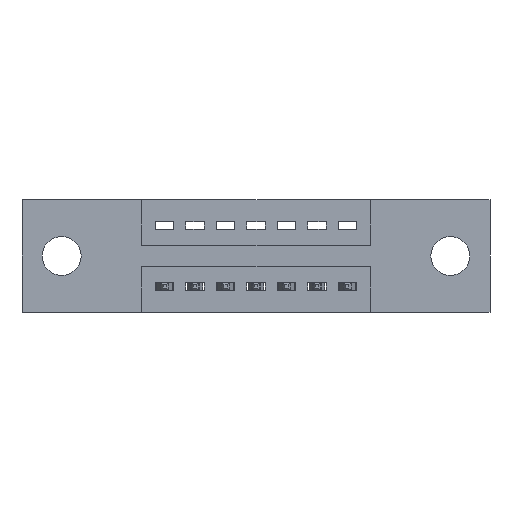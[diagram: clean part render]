
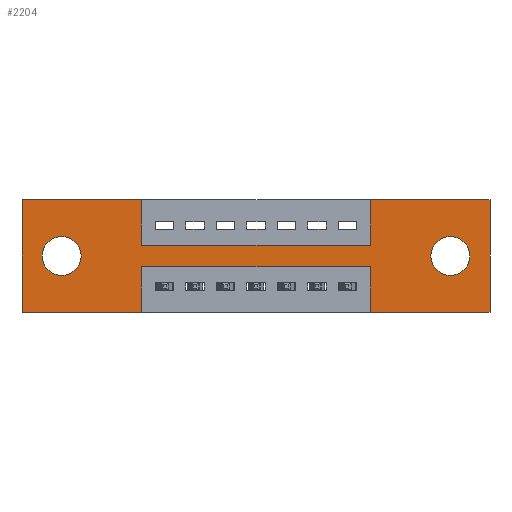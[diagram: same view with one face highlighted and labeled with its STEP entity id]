
A CAD part, front view. The second image highlights one B-rep face of the part: STEP entity #2204.
In plain terms, the highlighted planar face has unit normal (0, -1, 0).
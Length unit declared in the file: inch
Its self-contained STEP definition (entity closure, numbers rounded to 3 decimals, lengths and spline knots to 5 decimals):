
#175 = CARTESIAN_POINT ( 'NONE',  ( 0., 0., -0.37 ) ) ;
#200 = CARTESIAN_POINT ( 'NONE',  ( 0., 0., 0. ) ) ;
#263 = CARTESIAN_POINT ( 'NONE',  ( 0.3925, 0., -0.37 ) ) ;
#467 = CARTESIAN_POINT ( 'NONE',  ( 0., 0., -0.37 ) ) ;
#705 = VERTEX_POINT ( 'NONE', #1946 ) ;
#754 = EDGE_CURVE ( 'NONE', #2903, #5305, #3198, .T. ) ;
#755 = DIRECTION ( 'NONE',  ( 0., 0., -1. ) ) ;
#815 = ORIENTED_EDGE ( 'NONE', *, *, #8343, .F. ) ;
#854 = EDGE_CURVE ( 'NONE', #8996, #8657, #7049, .T. ) ;
#1015 = FACE_BOUND ( 'NONE', #9133, .T. ) ;
#1070 = CARTESIAN_POINT ( 'NONE',  ( 1.1425, 0., -0.22 ) ) ;
#1075 = AXIS2_PLACEMENT_3D ( 'NONE', #2217, #7555, #5308 ) ;
#1172 = ORIENTED_EDGE ( 'NONE', *, *, #2373, .F. ) ;
#1248 = VERTEX_POINT ( 'NONE', #8144 ) ;
#1264 = EDGE_CURVE ( 'NONE', #8352, #7169, #3689, .T. ) ;
#1525 = CIRCLE ( 'NONE', #3843, 0.064 ) ;
#1534 = DIRECTION ( 'NONE',  ( 0., 0., 1. ) ) ;
#1598 = LINE ( 'NONE', #7795, #9582 ) ;
#1729 = AXIS2_PLACEMENT_3D ( 'NONE', #3698, #6703, #9168 ) ;
#1784 = VECTOR ( 'NONE', #7000, 39.37008 ) ;
#1946 = CARTESIAN_POINT ( 'NONE',  ( 1.1425, 0., -0.15 ) ) ;
#2011 = DIRECTION ( 'NONE',  ( 1., 0., 0. ) ) ;
#2152 = PLANE ( 'NONE',  #1075 ) ;
#2199 = CARTESIAN_POINT ( 'NONE',  ( 1.405, 0., -0.121 ) ) ;
#2204 = ADVANCED_FACE ( 'NONE', ( #6083, #1015, #8509 ), #2152, .T. ) ;
#2217 = CARTESIAN_POINT ( 'NONE',  ( 0., 0., -0.37 ) ) ;
#2307 = EDGE_CURVE ( 'NONE', #7169, #2903, #1598, .T. ) ;
#2367 = DIRECTION ( 'NONE',  ( 0., 0., -1. ) ) ;
#2373 = EDGE_CURVE ( 'NONE', #5305, #9521, #9115, .T. ) ;
#2410 = EDGE_LOOP ( 'NONE', ( #6445, #5243, #4363, #8987, #815, #9466, #6175, #9647, #1172, #7229, #9069, #9988 ) ) ;
#2497 = CARTESIAN_POINT ( 'NONE',  ( 1.535, 0., 0. ) ) ;
#2546 = CARTESIAN_POINT ( 'NONE',  ( 1.405, 0., -0.249 ) ) ;
#2813 = CARTESIAN_POINT ( 'NONE',  ( 0.3925, 0., -0.37 ) ) ;
#2903 = VERTEX_POINT ( 'NONE', #9657 ) ;
#2953 = VERTEX_POINT ( 'NONE', #5676 ) ;
#3198 = LINE ( 'NONE', #3631, #4995 ) ;
#3357 = VERTEX_POINT ( 'NONE', #6620 ) ;
#3557 = CARTESIAN_POINT ( 'NONE',  ( 0.3925, 0., -0.22 ) ) ;
#3631 = CARTESIAN_POINT ( 'NONE',  ( 0., 0., 0. ) ) ;
#3689 = LINE ( 'NONE', #467, #6296 ) ;
#3698 = CARTESIAN_POINT ( 'NONE',  ( 0.13, 0., -0.185 ) ) ;
#3806 = EDGE_CURVE ( 'NONE', #2953, #8352, #5798, .T. ) ;
#3830 = CIRCLE ( 'NONE', #7728, 0.064 ) ;
#3843 = AXIS2_PLACEMENT_3D ( 'NONE', #6954, #7621, #755 ) ;
#3869 = LINE ( 'NONE', #5439, #1784 ) ;
#3884 = CARTESIAN_POINT ( 'NONE',  ( 1.535, 0., -0.37 ) ) ;
#4083 = VECTOR ( 'NONE', #8032, 39.37008 ) ;
#4292 = ORIENTED_EDGE ( 'NONE', *, *, #5644, .T. ) ;
#4363 = ORIENTED_EDGE ( 'NONE', *, *, #8855, .F. ) ;
#4454 = LINE ( 'NONE', #3557, #6737 ) ;
#4538 = DIRECTION ( 'NONE',  ( 1., 0., 0. ) ) ;
#4678 = DIRECTION ( 'NONE',  ( 0., 0., -1. ) ) ;
#4696 = EDGE_CURVE ( 'NONE', #9521, #705, #9186, .T. ) ;
#4995 = VECTOR ( 'NONE', #2011, 39.37008 ) ;
#5022 = ORIENTED_EDGE ( 'NONE', *, *, #9738, .T. ) ;
#5105 = DIRECTION ( 'NONE',  ( 0., 0., 1. ) ) ;
#5137 = DIRECTION ( 'NONE',  ( -1., 0., 0. ) ) ;
#5243 = ORIENTED_EDGE ( 'NONE', *, *, #7178, .F. ) ;
#5276 = CARTESIAN_POINT ( 'NONE',  ( 0.13, 0., -0.249 ) ) ;
#5305 = VERTEX_POINT ( 'NONE', #8476 ) ;
#5308 = DIRECTION ( 'NONE',  ( 0., 0., -1. ) ) ;
#5342 = EDGE_LOOP ( 'NONE', ( #9038, #4292 ) ) ;
#5385 = VERTEX_POINT ( 'NONE', #3884 ) ;
#5439 = CARTESIAN_POINT ( 'NONE',  ( 0., 0., -0.37 ) ) ;
#5533 = DIRECTION ( 'NONE',  ( 0., 1., 0. ) ) ;
#5644 = EDGE_CURVE ( 'NONE', #7117, #7827, #9764, .T. ) ;
#5646 = EDGE_CURVE ( 'NONE', #7827, #7117, #1525, .T. ) ;
#5676 = CARTESIAN_POINT ( 'NONE',  ( 0.3925, 0., -0.22 ) ) ;
#5688 = VERTEX_POINT ( 'NONE', #8698 ) ;
#5798 = LINE ( 'NONE', #2813, #6386 ) ;
#5833 = EDGE_CURVE ( 'NONE', #5385, #1248, #3869, .T. ) ;
#5989 = VERTEX_POINT ( 'NONE', #1070 ) ;
#6083 = FACE_BOUND ( 'NONE', #5342, .T. ) ;
#6175 = ORIENTED_EDGE ( 'NONE', *, *, #8043, .F. ) ;
#6296 = VECTOR ( 'NONE', #5137, 39.37008 ) ;
#6386 = VECTOR ( 'NONE', #9870, 39.37008 ) ;
#6388 = AXIS2_PLACEMENT_3D ( 'NONE', #9788, #5533, #8443 ) ;
#6427 = CARTESIAN_POINT ( 'NONE',  ( 0.3925, 0., -0.15 ) ) ;
#6445 = ORIENTED_EDGE ( 'NONE', *, *, #3806, .F. ) ;
#6493 = CARTESIAN_POINT ( 'NONE',  ( 0.13, 0., -0.185 ) ) ;
#6524 = CARTESIAN_POINT ( 'NONE',  ( 1.1425, 0., 0. ) ) ;
#6620 = CARTESIAN_POINT ( 'NONE',  ( 1.535, 0., 0. ) ) ;
#6703 = DIRECTION ( 'NONE',  ( 0., 1., 0. ) ) ;
#6737 = VECTOR ( 'NONE', #8962, 39.37008 ) ;
#6921 = CARTESIAN_POINT ( 'NONE',  ( 1.1425, 0., -0.37 ) ) ;
#6928 = LINE ( 'NONE', #6921, #9862 ) ;
#6954 = CARTESIAN_POINT ( 'NONE',  ( 1.405, 0., -0.185 ) ) ;
#7000 = DIRECTION ( 'NONE',  ( -1., 0., 0. ) ) ;
#7049 = CIRCLE ( 'NONE', #1729, 0.064 ) ;
#7060 = CARTESIAN_POINT ( 'NONE',  ( 0.3925, 0., 0. ) ) ;
#7117 = VERTEX_POINT ( 'NONE', #2546 ) ;
#7169 = VERTEX_POINT ( 'NONE', #175 ) ;
#7178 = EDGE_CURVE ( 'NONE', #5989, #2953, #4454, .T. ) ;
#7191 = VECTOR ( 'NONE', #2367, 39.37008 ) ;
#7229 = ORIENTED_EDGE ( 'NONE', *, *, #754, .F. ) ;
#7555 = DIRECTION ( 'NONE',  ( 0., -1., 0. ) ) ;
#7621 = DIRECTION ( 'NONE',  ( 0., 1., 0. ) ) ;
#7728 = AXIS2_PLACEMENT_3D ( 'NONE', #6493, #8081, #5105 ) ;
#7742 = ORIENTED_EDGE ( 'NONE', *, *, #854, .T. ) ;
#7758 = EDGE_CURVE ( 'NONE', #5688, #3357, #8449, .T. ) ;
#7795 = CARTESIAN_POINT ( 'NONE',  ( 0., 0., 0. ) ) ;
#7827 = VERTEX_POINT ( 'NONE', #2199 ) ;
#7830 = LINE ( 'NONE', #6524, #8794 ) ;
#8032 = DIRECTION ( 'NONE',  ( 1., 0., 0. ) ) ;
#8043 = EDGE_CURVE ( 'NONE', #705, #5688, #7830, .T. ) ;
#8081 = DIRECTION ( 'NONE',  ( 0., 1., 0. ) ) ;
#8144 = CARTESIAN_POINT ( 'NONE',  ( 1.1425, 0., -0.37 ) ) ;
#8343 = EDGE_CURVE ( 'NONE', #3357, #5385, #9268, .T. ) ;
#8352 = VERTEX_POINT ( 'NONE', #263 ) ;
#8443 = DIRECTION ( 'NONE',  ( 0., 0., -1. ) ) ;
#8449 = LINE ( 'NONE', #200, #4083 ) ;
#8476 = CARTESIAN_POINT ( 'NONE',  ( 0.3925, 0., 0. ) ) ;
#8509 = FACE_OUTER_BOUND ( 'NONE', #2410, .T. ) ;
#8608 = CARTESIAN_POINT ( 'NONE',  ( 0.13, 0., -0.121 ) ) ;
#8657 = VERTEX_POINT ( 'NONE', #5276 ) ;
#8698 = CARTESIAN_POINT ( 'NONE',  ( 1.1425, 0., 0. ) ) ;
#8735 = DIRECTION ( 'NONE',  ( 0., 0., 1. ) ) ;
#8752 = VECTOR ( 'NONE', #4678, 39.37008 ) ;
#8794 = VECTOR ( 'NONE', #9698, 39.37008 ) ;
#8855 = EDGE_CURVE ( 'NONE', #1248, #5989, #6928, .T. ) ;
#8962 = DIRECTION ( 'NONE',  ( -1., 0., 0. ) ) ;
#8987 = ORIENTED_EDGE ( 'NONE', *, *, #5833, .F. ) ;
#8996 = VERTEX_POINT ( 'NONE', #8608 ) ;
#9038 = ORIENTED_EDGE ( 'NONE', *, *, #5646, .T. ) ;
#9069 = ORIENTED_EDGE ( 'NONE', *, *, #2307, .F. ) ;
#9115 = LINE ( 'NONE', #7060, #8752 ) ;
#9133 = EDGE_LOOP ( 'NONE', ( #7742, #5022 ) ) ;
#9168 = DIRECTION ( 'NONE',  ( 0., 0., 1. ) ) ;
#9185 = CARTESIAN_POINT ( 'NONE',  ( 0.3925, 0., -0.15 ) ) ;
#9186 = LINE ( 'NONE', #9185, #9524 ) ;
#9268 = LINE ( 'NONE', #2497, #7191 ) ;
#9466 = ORIENTED_EDGE ( 'NONE', *, *, #7758, .F. ) ;
#9521 = VERTEX_POINT ( 'NONE', #6427 ) ;
#9524 = VECTOR ( 'NONE', #4538, 39.37008 ) ;
#9582 = VECTOR ( 'NONE', #1534, 39.37008 ) ;
#9647 = ORIENTED_EDGE ( 'NONE', *, *, #4696, .F. ) ;
#9657 = CARTESIAN_POINT ( 'NONE',  ( 0., 0., 0. ) ) ;
#9698 = DIRECTION ( 'NONE',  ( 0., 0., 1. ) ) ;
#9738 = EDGE_CURVE ( 'NONE', #8657, #8996, #3830, .T. ) ;
#9764 = CIRCLE ( 'NONE', #6388, 0.064 ) ;
#9788 = CARTESIAN_POINT ( 'NONE',  ( 1.405, 0., -0.185 ) ) ;
#9862 = VECTOR ( 'NONE', #8735, 39.37008 ) ;
#9870 = DIRECTION ( 'NONE',  ( 0., 0., -1. ) ) ;
#9988 = ORIENTED_EDGE ( 'NONE', *, *, #1264, .F. ) ;
